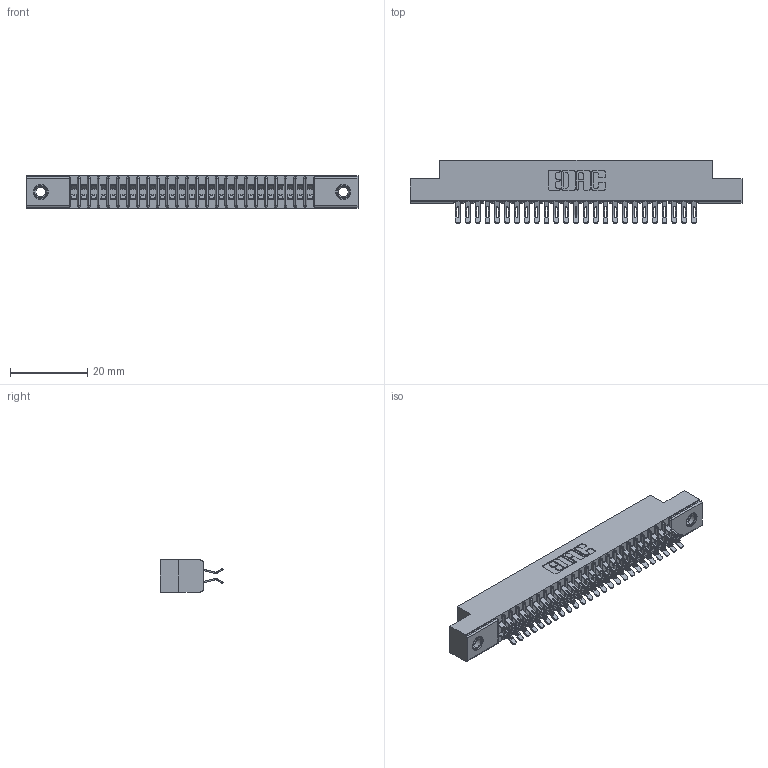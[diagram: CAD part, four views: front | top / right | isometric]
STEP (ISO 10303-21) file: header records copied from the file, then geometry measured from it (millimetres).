
FILE_DESCRIPTION (( 'STEP AP203' ), '1' );
FILE_NAME ('391-050-555-207.STEP', '2018-08-09T05:21:45', ( '' ), ( '' ), 'SwSTEP 2.0', 'SolidWorks 2016', '' );
FILE_SCHEMA (( 'CONFIG_CONTROL_DESIGN' ));
Length unit declared in the file: inch
Products named in the file (4): 345-250-001_345-250-005-103; 391-050-555-207; 341 Part_.156 (3.96) Dia Mounting Holes; 341-292-001_341-292-155
Assembly tree (53 placements, depth 2):
  391-050-555-207
    341 Part_.156 (3.96) Dia Mounting Holes
    341-292-001_341-292-155  x50
    345-250-001_345-250-005-103  x2
Bounding box: 85.72 x 16.31 x 8.38 mm (x, y, z)
Volume: 4922.3 mm3; surface area: 10864.5 mm2
Topology: 53 solids, 53 shells, 4076 faces, 12127 edges, 7890 vertices
Faces by surface type: plane 2200, cylinder 1760, sphere 52, torus 52, cone 12
Entity records: 34175 total; most frequent: CARTESIAN_POINT 5680, ORIENTED_EDGE 5626, DIRECTION 5525, EDGE_CURVE 2813, VECTOR 2235, LINE 2235, VERTEX_POINT 1784, AXIS2_PLACEMENT_3D 1645
